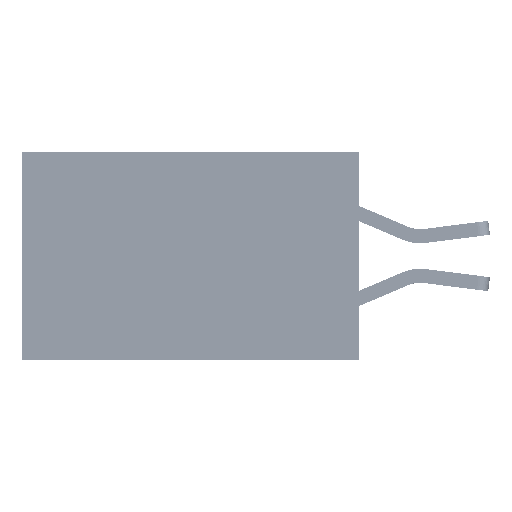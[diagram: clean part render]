
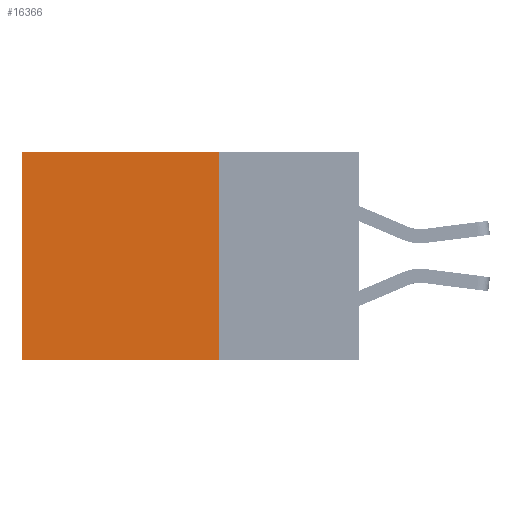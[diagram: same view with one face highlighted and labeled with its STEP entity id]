
A CAD part, left-side view. The second image highlights one B-rep face of the part: STEP entity #16366.
In plain terms, the highlighted planar face has unit normal (-1, 0, 0).
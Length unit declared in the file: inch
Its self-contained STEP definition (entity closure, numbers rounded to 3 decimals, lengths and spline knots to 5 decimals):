
#894 = FACE_OUTER_BOUND ( 'NONE', #19486, .T. ) ;
#1409 = VECTOR ( 'NONE', #38299, 39.37008 ) ;
#9280 = DIRECTION ( 'NONE',  ( 0., 0., -1. ) ) ;
#9366 = ORIENTED_EDGE ( 'NONE', *, *, #17234, .T. ) ;
#10285 = AXIS2_PLACEMENT_3D ( 'NONE', #33778, #30018, #9280 ) ;
#11616 = ORIENTED_EDGE ( 'NONE', *, *, #47607, .T. ) ;
#15973 = CARTESIAN_POINT ( 'NONE',  ( 0.2875, 0.25, -0.37 ) ) ;
#16062 = VERTEX_POINT ( 'NONE', #52275 ) ;
#16366 = ADVANCED_FACE ( 'NONE', ( #894 ), #17375, .F. ) ;
#17058 = CARTESIAN_POINT ( 'NONE',  ( 0.2875, 0.25, -0.37 ) ) ;
#17234 = EDGE_CURVE ( 'NONE', #16062, #40845, #22362, .T. ) ;
#17375 = PLANE ( 'NONE',  #10285 ) ;
#19486 = EDGE_LOOP ( 'NONE', ( #9366, #41849, #49681, #11616 ) ) ;
#20646 = VERTEX_POINT ( 'NONE', #15973 ) ;
#21237 = LINE ( 'NONE', #41964, #24503 ) ;
#22095 = DIRECTION ( 'NONE',  ( 0., 0., -1. ) ) ;
#22362 = LINE ( 'NONE', #26391, #47354 ) ;
#24503 = VECTOR ( 'NONE', #36847, 39.37008 ) ;
#25189 = VERTEX_POINT ( 'NONE', #44038 ) ;
#26391 = CARTESIAN_POINT ( 'NONE',  ( 0.2875, 0.6, 0. ) ) ;
#28982 = LINE ( 'NONE', #49724, #30320 ) ;
#30018 = DIRECTION ( 'NONE',  ( 1., 0., 0. ) ) ;
#30320 = VECTOR ( 'NONE', #49190, 39.37008 ) ;
#33778 = CARTESIAN_POINT ( 'NONE',  ( 0.2875, 0.25, 0. ) ) ;
#36392 = EDGE_CURVE ( 'NONE', #25189, #20646, #21237, .T. ) ;
#36847 = DIRECTION ( 'NONE',  ( 0., 0., -1. ) ) ;
#37488 = LINE ( 'NONE', #17058, #1409 ) ;
#38299 = DIRECTION ( 'NONE',  ( 0., 1., 0. ) ) ;
#40845 = VERTEX_POINT ( 'NONE', #45697 ) ;
#41849 = ORIENTED_EDGE ( 'NONE', *, *, #52655, .F. ) ;
#41964 = CARTESIAN_POINT ( 'NONE',  ( 0.2875, 0.25, 0. ) ) ;
#44038 = CARTESIAN_POINT ( 'NONE',  ( 0.2875, 0.25, 0. ) ) ;
#45697 = CARTESIAN_POINT ( 'NONE',  ( 0.2875, 0.6, -0.37 ) ) ;
#47354 = VECTOR ( 'NONE', #22095, 39.37008 ) ;
#47607 = EDGE_CURVE ( 'NONE', #25189, #16062, #28982, .T. ) ;
#49190 = DIRECTION ( 'NONE',  ( 0., 1., 0. ) ) ;
#49681 = ORIENTED_EDGE ( 'NONE', *, *, #36392, .F. ) ;
#49724 = CARTESIAN_POINT ( 'NONE',  ( 0.2875, 0.25, 0. ) ) ;
#52275 = CARTESIAN_POINT ( 'NONE',  ( 0.2875, 0.6, 0. ) ) ;
#52655 = EDGE_CURVE ( 'NONE', #20646, #40845, #37488, .T. ) ;
